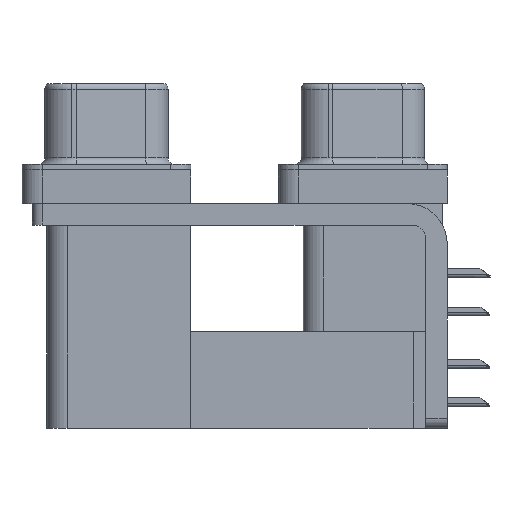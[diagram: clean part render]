
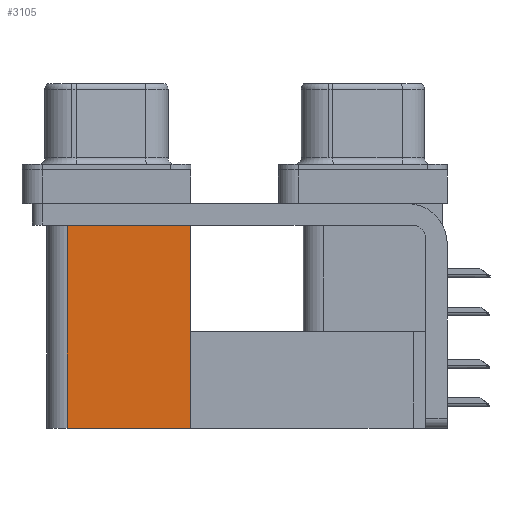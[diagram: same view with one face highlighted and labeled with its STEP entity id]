
A CAD part, left-side view. The second image highlights one B-rep face of the part: STEP entity #3105.
In plain terms, the highlighted planar face has unit normal (-1, 0, 0).
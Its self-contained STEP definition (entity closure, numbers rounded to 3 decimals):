
#1016 = LINE ( 'NONE', #10717, #3383 ) ;
#1175 = DIRECTION ( 'NONE',  ( 0., 0., 1. ) ) ;
#1402 = VERTEX_POINT ( 'NONE', #16755 ) ;
#2008 = EDGE_CURVE ( 'NONE', #4883, #1402, #5571, .T. ) ;
#2855 = CARTESIAN_POINT ( 'NONE',  ( 3.765, 21.975, -19.2 ) ) ;
#3105 = ADVANCED_FACE ( 'NONE', ( #19907 ), #7825, .F. ) ;
#3209 = DIRECTION ( 'NONE',  ( 0., 1., 0. ) ) ;
#3383 = VECTOR ( 'NONE', #1175, 1000. ) ;
#3646 = CARTESIAN_POINT ( 'NONE',  ( 3.765, 21.975, -19.2 ) ) ;
#4883 = VERTEX_POINT ( 'NONE', #3646 ) ;
#5571 = LINE ( 'NONE', #2855, #29891 ) ;
#5781 = CARTESIAN_POINT ( 'NONE',  ( 3.765, 12.775, -19.2 ) ) ;
#7454 = DIRECTION ( 'NONE',  ( 0., 1., 0. ) ) ;
#7825 = PLANE ( 'NONE',  #11400 ) ;
#8026 = CARTESIAN_POINT ( 'NONE',  ( 3.765, 12.775, -2.5 ) ) ;
#8439 = ORIENTED_EDGE ( 'NONE', *, *, #13680, .F. ) ;
#9544 = VERTEX_POINT ( 'NONE', #5781 ) ;
#9823 = LINE ( 'NONE', #29208, #27925 ) ;
#10717 = CARTESIAN_POINT ( 'NONE',  ( 3.765, 12.775, -19.2 ) ) ;
#11400 = AXIS2_PLACEMENT_3D ( 'NONE', #15293, #25000, #3209 ) ;
#11412 = LINE ( 'NONE', #19210, #13694 ) ;
#13022 = DIRECTION ( 'NONE',  ( 0., 0., 1. ) ) ;
#13406 = EDGE_CURVE ( 'NONE', #23608, #1402, #11412, .T. ) ;
#13680 = EDGE_CURVE ( 'NONE', #9544, #4883, #9823, .T. ) ;
#13694 = VECTOR ( 'NONE', #14423, 1000. ) ;
#14423 = DIRECTION ( 'NONE',  ( 0., 1., 0. ) ) ;
#15293 = CARTESIAN_POINT ( 'NONE',  ( 3.765, 12.775, -19.2 ) ) ;
#16755 = CARTESIAN_POINT ( 'NONE',  ( 3.765, 21.975, -2.5 ) ) ;
#19210 = CARTESIAN_POINT ( 'NONE',  ( 3.765, 12.775, -2.5 ) ) ;
#19907 = FACE_OUTER_BOUND ( 'NONE', #22912, .T. ) ;
#20605 = EDGE_CURVE ( 'NONE', #9544, #23608, #1016, .T. ) ;
#20765 = ORIENTED_EDGE ( 'NONE', *, *, #2008, .F. ) ;
#21930 = ORIENTED_EDGE ( 'NONE', *, *, #13406, .T. ) ;
#22912 = EDGE_LOOP ( 'NONE', ( #21930, #20765, #8439, #31304 ) ) ;
#23608 = VERTEX_POINT ( 'NONE', #8026 ) ;
#25000 = DIRECTION ( 'NONE',  ( 1., 0., 0. ) ) ;
#27925 = VECTOR ( 'NONE', #7454, 1000. ) ;
#29208 = CARTESIAN_POINT ( 'NONE',  ( 3.765, 12.775, -19.2 ) ) ;
#29891 = VECTOR ( 'NONE', #13022, 1000. ) ;
#31304 = ORIENTED_EDGE ( 'NONE', *, *, #20605, .T. ) ;
